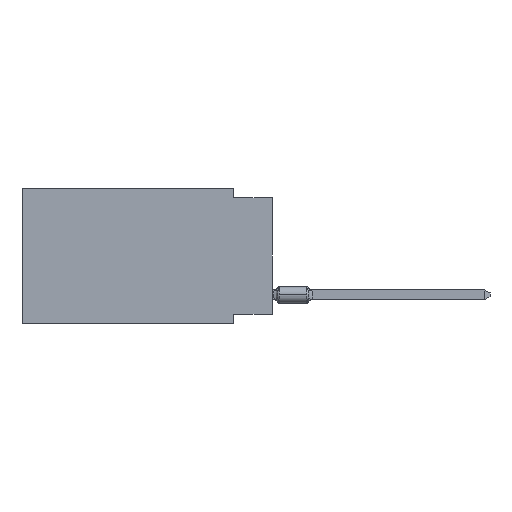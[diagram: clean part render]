
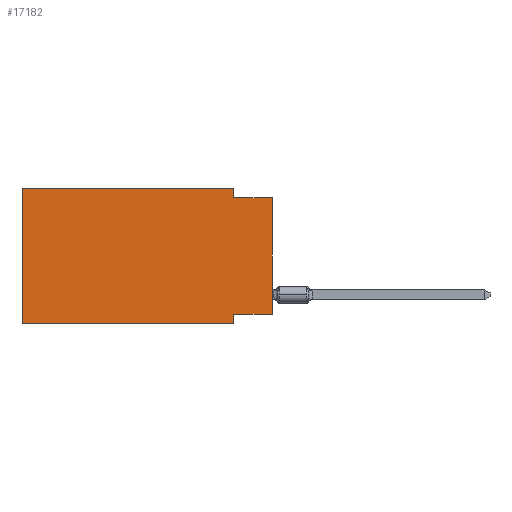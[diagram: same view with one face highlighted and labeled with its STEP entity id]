
A CAD part, left-side view. The second image highlights one B-rep face of the part: STEP entity #17182.
In plain terms, the highlighted planar face has unit normal (-1, 0, 0).
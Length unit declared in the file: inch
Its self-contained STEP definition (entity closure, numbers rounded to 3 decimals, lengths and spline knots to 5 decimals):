
#860 = LINE ( 'NONE', #16877, #21519 ) ;
#1185 = ORIENTED_EDGE ( 'NONE', *, *, #35075, .T. ) ;
#1421 = ORIENTED_EDGE ( 'NONE', *, *, #26493, .F. ) ;
#1810 = DIRECTION ( 'NONE',  ( 0., 1., 0. ) ) ;
#1908 = VECTOR ( 'NONE', #21053, 39.37008 ) ;
#2097 = VERTEX_POINT ( 'NONE', #15959 ) ;
#2371 = LINE ( 'NONE', #18220, #1908 ) ;
#3907 = EDGE_CURVE ( 'NONE', #2097, #25282, #18061, .T. ) ;
#4299 = LINE ( 'NONE', #12494, #13794 ) ;
#4655 = LINE ( 'NONE', #20266, #6553 ) ;
#4774 = DIRECTION ( 'NONE',  ( 0., -1., 0. ) ) ;
#5365 = VERTEX_POINT ( 'NONE', #24521 ) ;
#5480 = CARTESIAN_POINT ( 'NONE',  ( 0., 0.645, 0. ) ) ;
#5553 = PLANE ( 'NONE',  #19854 ) ;
#5625 = VECTOR ( 'NONE', #21312, 39.37008 ) ;
#6144 = CARTESIAN_POINT ( 'NONE',  ( 0., 0.645, 0. ) ) ;
#6304 = ORIENTED_EDGE ( 'NONE', *, *, #33839, .F. ) ;
#6445 = VECTOR ( 'NONE', #4774, 39.37008 ) ;
#6553 = VECTOR ( 'NONE', #31617, 39.37008 ) ;
#6625 = EDGE_CURVE ( 'NONE', #5365, #16465, #4655, .T. ) ;
#7359 = VECTOR ( 'NONE', #12557, 39.37008 ) ;
#10125 = EDGE_CURVE ( 'NONE', #20001, #17423, #20963, .T. ) ;
#11542 = DIRECTION ( 'NONE',  ( 0., -1., 0. ) ) ;
#12494 = CARTESIAN_POINT ( 'NONE',  ( 0., 0., -0.325 ) ) ;
#12557 = DIRECTION ( 'NONE',  ( 0., 0., -1. ) ) ;
#13547 = DIRECTION ( 'NONE',  ( 0., 0., -1. ) ) ;
#13794 = VECTOR ( 'NONE', #1810, 39.37008 ) ;
#15049 = LINE ( 'NONE', #25880, #7359 ) ;
#15959 = CARTESIAN_POINT ( 'NONE',  ( 0., 0.1, -0.325 ) ) ;
#16171 = LINE ( 'NONE', #5480, #5625 ) ;
#16241 = DIRECTION ( 'NONE',  ( 1., 0., 0. ) ) ;
#16465 = VERTEX_POINT ( 'NONE', #25360 ) ;
#16877 = CARTESIAN_POINT ( 'NONE',  ( 0., 0., -0.025 ) ) ;
#17182 = ADVANCED_FACE ( 'NONE', ( #27608 ), #5553, .F. ) ;
#17423 = VERTEX_POINT ( 'NONE', #23666 ) ;
#18061 = LINE ( 'NONE', #31198, #31520 ) ;
#18220 = CARTESIAN_POINT ( 'NONE',  ( 0., 0.645, -0.35 ) ) ;
#18352 = CARTESIAN_POINT ( 'NONE',  ( 0., 0.1, -0.35 ) ) ;
#19646 = ORIENTED_EDGE ( 'NONE', *, *, #6625, .T. ) ;
#19854 = AXIS2_PLACEMENT_3D ( 'NONE', #21738, #16241, #32570 ) ;
#20001 = VERTEX_POINT ( 'NONE', #6144 ) ;
#20266 = CARTESIAN_POINT ( 'NONE',  ( 0., 0., 0. ) ) ;
#20663 = ORIENTED_EDGE ( 'NONE', *, *, #10125, .F. ) ;
#20963 = LINE ( 'NONE', #29139, #6445 ) ;
#21053 = DIRECTION ( 'NONE',  ( 0., -1., 0. ) ) ;
#21312 = DIRECTION ( 'NONE',  ( 0., 0., 1. ) ) ;
#21519 = VECTOR ( 'NONE', #11542, 39.37008 ) ;
#21563 = VERTEX_POINT ( 'NONE', #26950 ) ;
#21738 = CARTESIAN_POINT ( 'NONE',  ( 0., 0.645, 0. ) ) ;
#23666 = CARTESIAN_POINT ( 'NONE',  ( 0., 0.1, 0. ) ) ;
#24521 = CARTESIAN_POINT ( 'NONE',  ( 0., 0., -0.325 ) ) ;
#25282 = VERTEX_POINT ( 'NONE', #18352 ) ;
#25360 = CARTESIAN_POINT ( 'NONE',  ( 0., 0., -0.025 ) ) ;
#25880 = CARTESIAN_POINT ( 'NONE',  ( 0., 0.1, 0. ) ) ;
#26493 = EDGE_CURVE ( 'NONE', #17423, #32784, #15049, .T. ) ;
#26950 = CARTESIAN_POINT ( 'NONE',  ( 0., 0.645, -0.35 ) ) ;
#27389 = ORIENTED_EDGE ( 'NONE', *, *, #3907, .F. ) ;
#27423 = EDGE_LOOP ( 'NONE', ( #19646, #34415, #1421, #20663, #33448, #1185, #27389, #6304 ) ) ;
#27608 = FACE_OUTER_BOUND ( 'NONE', #27423, .T. ) ;
#29030 = EDGE_CURVE ( 'NONE', #21563, #20001, #16171, .T. ) ;
#29139 = CARTESIAN_POINT ( 'NONE',  ( 0., 0.645, 0. ) ) ;
#29227 = EDGE_CURVE ( 'NONE', #32784, #16465, #860, .T. ) ;
#29510 = CARTESIAN_POINT ( 'NONE',  ( 0., 0.1, -0.025 ) ) ;
#31198 = CARTESIAN_POINT ( 'NONE',  ( 0., 0.1, -0.35 ) ) ;
#31520 = VECTOR ( 'NONE', #13547, 39.37008 ) ;
#31617 = DIRECTION ( 'NONE',  ( 0., 0., 1. ) ) ;
#32570 = DIRECTION ( 'NONE',  ( 0., 0., -1. ) ) ;
#32784 = VERTEX_POINT ( 'NONE', #29510 ) ;
#33448 = ORIENTED_EDGE ( 'NONE', *, *, #29030, .F. ) ;
#33839 = EDGE_CURVE ( 'NONE', #5365, #2097, #4299, .T. ) ;
#34415 = ORIENTED_EDGE ( 'NONE', *, *, #29227, .F. ) ;
#35075 = EDGE_CURVE ( 'NONE', #21563, #25282, #2371, .T. ) ;
